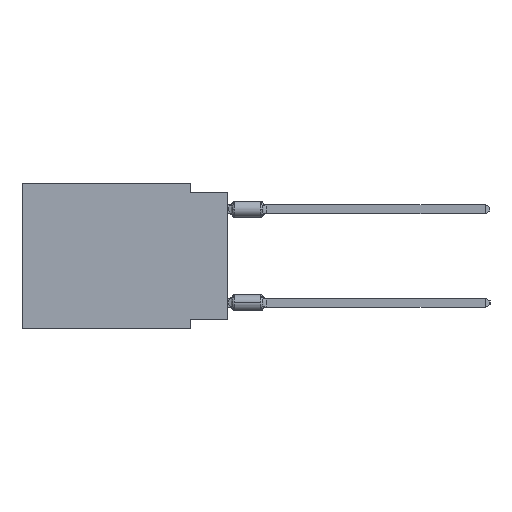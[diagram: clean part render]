
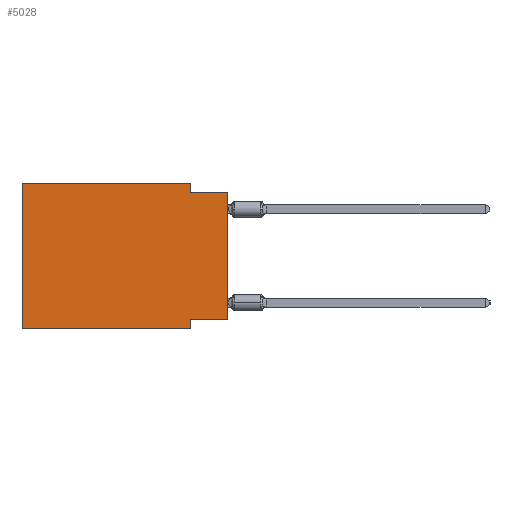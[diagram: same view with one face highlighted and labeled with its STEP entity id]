
A CAD part, left-side view. The second image highlights one B-rep face of the part: STEP entity #5028.
In plain terms, the highlighted planar face has unit normal (-1, 0, 0).
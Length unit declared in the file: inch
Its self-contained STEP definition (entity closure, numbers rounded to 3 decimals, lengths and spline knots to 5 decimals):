
#1476 = CARTESIAN_POINT ( 'NONE',  ( 0., 0.1, 0. ) ) ;
#1752 = LINE ( 'NONE', #38172, #4860 ) ;
#4397 = DIRECTION ( 'NONE',  ( 0., 0., -1. ) ) ;
#4437 = ORIENTED_EDGE ( 'NONE', *, *, #7745, .T. ) ;
#4596 = VERTEX_POINT ( 'NONE', #25584 ) ;
#4601 = EDGE_CURVE ( 'NONE', #46391, #19985, #18132, .T. ) ;
#4860 = VECTOR ( 'NONE', #18333, 39.37008 ) ;
#5028 = ADVANCED_FACE ( 'NONE', ( #6192 ), #41630, .F. ) ;
#5997 = ORIENTED_EDGE ( 'NONE', *, *, #41224, .F. ) ;
#6123 = EDGE_CURVE ( 'NONE', #45576, #4596, #36172, .T. ) ;
#6192 = FACE_OUTER_BOUND ( 'NONE', #6282, .T. ) ;
#6282 = EDGE_LOOP ( 'NONE', ( #43175, #39776, #8812, #45736, #5997, #4437, #32688, #18742 ) ) ;
#7167 = CARTESIAN_POINT ( 'NONE',  ( 0., 0.55, -0.39 ) ) ;
#7321 = LINE ( 'NONE', #26387, #19314 ) ;
#7443 = LINE ( 'NONE', #31491, #30333 ) ;
#7745 = EDGE_CURVE ( 'NONE', #24866, #29534, #7321, .T. ) ;
#8812 = ORIENTED_EDGE ( 'NONE', *, *, #41982, .F. ) ;
#9608 = LINE ( 'NONE', #26520, #27597 ) ;
#10523 = LINE ( 'NONE', #38833, #31068 ) ;
#11034 = DIRECTION ( 'NONE',  ( 0., -1., 0. ) ) ;
#14178 = CARTESIAN_POINT ( 'NONE',  ( 0., 0., -0.365 ) ) ;
#15114 = CARTESIAN_POINT ( 'NONE',  ( 0., 0.1, 0. ) ) ;
#18132 = LINE ( 'NONE', #14178, #50124 ) ;
#18333 = DIRECTION ( 'NONE',  ( 0., -1., 0. ) ) ;
#18742 = ORIENTED_EDGE ( 'NONE', *, *, #4601, .F. ) ;
#19314 = VECTOR ( 'NONE', #11034, 39.37008 ) ;
#19985 = VERTEX_POINT ( 'NONE', #23518 ) ;
#21530 = DIRECTION ( 'NONE',  ( 0., 0., -1. ) ) ;
#21812 = CARTESIAN_POINT ( 'NONE',  ( 0., 0.55, 0. ) ) ;
#22733 = VECTOR ( 'NONE', #36688, 39.37008 ) ;
#23518 = CARTESIAN_POINT ( 'NONE',  ( 0., 0.1, -0.365 ) ) ;
#24866 = VERTEX_POINT ( 'NONE', #7167 ) ;
#25584 = CARTESIAN_POINT ( 'NONE',  ( 0., 0., -0.025 ) ) ;
#26228 = CARTESIAN_POINT ( 'NONE',  ( 0., 0.1, -0.39 ) ) ;
#26387 = CARTESIAN_POINT ( 'NONE',  ( 0., 0.55, -0.39 ) ) ;
#26520 = CARTESIAN_POINT ( 'NONE',  ( 0., 0.1, -0.39 ) ) ;
#27597 = VECTOR ( 'NONE', #42625, 39.37008 ) ;
#29534 = VERTEX_POINT ( 'NONE', #26228 ) ;
#29792 = DIRECTION ( 'NONE',  ( 0., 1., 0. ) ) ;
#30333 = VECTOR ( 'NONE', #43648, 39.37008 ) ;
#31068 = VECTOR ( 'NONE', #50716, 39.37008 ) ;
#31491 = CARTESIAN_POINT ( 'NONE',  ( 0., 0., 0. ) ) ;
#32688 = ORIENTED_EDGE ( 'NONE', *, *, #46641, .F. ) ;
#33395 = VERTEX_POINT ( 'NONE', #15114 ) ;
#34087 = VERTEX_POINT ( 'NONE', #38795 ) ;
#35732 = CARTESIAN_POINT ( 'NONE',  ( 0., 0.1, -0.025 ) ) ;
#36069 = VECTOR ( 'NONE', #4397, 39.37008 ) ;
#36172 = LINE ( 'NONE', #44112, #22733 ) ;
#36688 = DIRECTION ( 'NONE',  ( 0., -1., 0. ) ) ;
#37403 = DIRECTION ( 'NONE',  ( 1., 0., 0. ) ) ;
#37648 = LINE ( 'NONE', #1476, #36069 ) ;
#38172 = CARTESIAN_POINT ( 'NONE',  ( 0., 0.55, 0. ) ) ;
#38795 = CARTESIAN_POINT ( 'NONE',  ( 0., 0.55, 0. ) ) ;
#38833 = CARTESIAN_POINT ( 'NONE',  ( 0., 0.55, 0. ) ) ;
#38851 = EDGE_CURVE ( 'NONE', #46391, #4596, #7443, .T. ) ;
#39776 = ORIENTED_EDGE ( 'NONE', *, *, #6123, .F. ) ;
#41224 = EDGE_CURVE ( 'NONE', #24866, #34087, #10523, .T. ) ;
#41630 = PLANE ( 'NONE',  #50982 ) ;
#41982 = EDGE_CURVE ( 'NONE', #33395, #45576, #37648, .T. ) ;
#42075 = EDGE_CURVE ( 'NONE', #34087, #33395, #1752, .T. ) ;
#42625 = DIRECTION ( 'NONE',  ( 0., 0., -1. ) ) ;
#43175 = ORIENTED_EDGE ( 'NONE', *, *, #38851, .T. ) ;
#43648 = DIRECTION ( 'NONE',  ( 0., 0., 1. ) ) ;
#44112 = CARTESIAN_POINT ( 'NONE',  ( 0., 0., -0.025 ) ) ;
#45576 = VERTEX_POINT ( 'NONE', #35732 ) ;
#45736 = ORIENTED_EDGE ( 'NONE', *, *, #42075, .F. ) ;
#46391 = VERTEX_POINT ( 'NONE', #47200 ) ;
#46641 = EDGE_CURVE ( 'NONE', #19985, #29534, #9608, .T. ) ;
#47200 = CARTESIAN_POINT ( 'NONE',  ( 0., 0., -0.365 ) ) ;
#50124 = VECTOR ( 'NONE', #29792, 39.37008 ) ;
#50716 = DIRECTION ( 'NONE',  ( 0., 0., 1. ) ) ;
#50982 = AXIS2_PLACEMENT_3D ( 'NONE', #21812, #37403, #21530 ) ;
